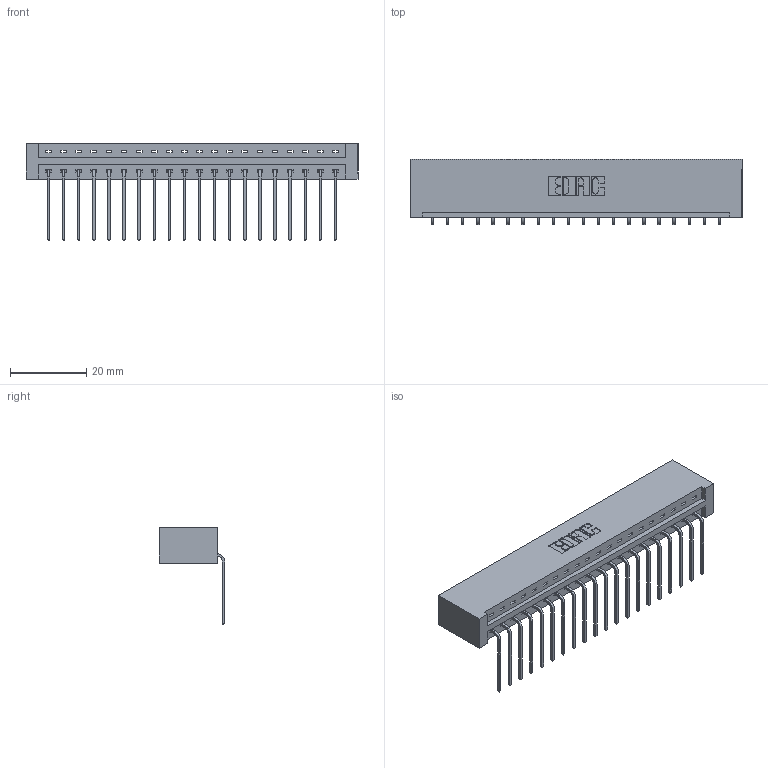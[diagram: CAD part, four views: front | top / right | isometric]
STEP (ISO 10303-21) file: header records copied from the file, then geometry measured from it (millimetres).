
FILE_DESCRIPTION (( 'STEP AP203' ), '1' );
FILE_NAME ('387-020-559-101.STEP', '2018-09-14T00:33:35', ( '' ), ( '' ), 'SwSTEP 2.0', 'SolidWorks 2016', '' );
FILE_SCHEMA (( 'CONFIG_CONTROL_DESIGN' ));
Length unit declared in the file: inch
Products named in the file (3): 337 Part_No Mounting Lugs; 345-292-001_558 559 Tail - 1; 387-020-559-101
Assembly tree (21 placements, depth 2):
  387-020-559-101
    337 Part_No Mounting Lugs
    345-292-001_558 559 Tail - 1  x20
Bounding box: 87.12 x 17.09 x 25.53 mm (x, y, z)
Volume: 9584.9 mm3; surface area: 10173.3 mm2
Topology: 21 solids, 21 shells, 1386 faces, 4167 edges, 2750 vertices
Faces by surface type: plane 1026, cylinder 360
Entity records: 17519 total; most frequent: CARTESIAN_POINT 3058, ORIENTED_EDGE 3014, DIRECTION 2611, EDGE_CURVE 1507, VECTOR 1387, LINE 1387, VERTEX_POINT 1002, AXIS2_PLACEMENT_3D 612
